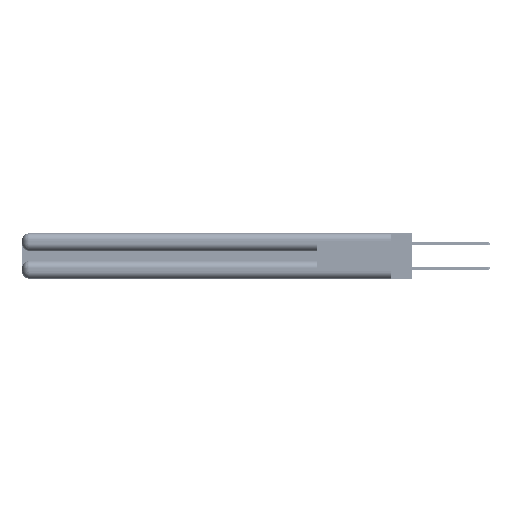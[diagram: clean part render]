
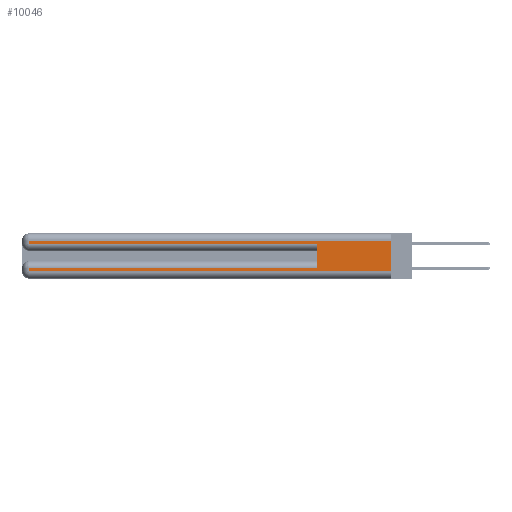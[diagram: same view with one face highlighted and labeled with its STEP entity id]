
A CAD part, left-side view. The second image highlights one B-rep face of the part: STEP entity #10046.
In plain terms, the highlighted planar face has unit normal (-1, 0, 0).
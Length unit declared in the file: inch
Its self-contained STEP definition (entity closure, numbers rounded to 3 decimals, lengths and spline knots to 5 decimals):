
#1455 = VERTEX_POINT ( 'NONE', #49478 ) ;
#1917 = DIRECTION ( 'NONE',  ( 0., 1., 0. ) ) ;
#2468 = CARTESIAN_POINT ( 'NONE',  ( 0., 0.6, 0.285 ) ) ;
#3749 = ORIENTED_EDGE ( 'NONE', *, *, #15448, .T. ) ;
#4022 = VECTOR ( 'NONE', #41665, 39.37008 ) ;
#4576 = EDGE_CURVE ( 'NONE', #1455, #8995, #44845, .T. ) ;
#5331 = LINE ( 'NONE', #37475, #4022 ) ;
#8507 = CARTESIAN_POINT ( 'NONE',  ( 0., 0., 0.06 ) ) ;
#8995 = VERTEX_POINT ( 'NONE', #20734 ) ;
#10046 = ADVANCED_FACE ( 'NONE', ( #35135 ), #47172, .F. ) ;
#10300 = ORIENTED_EDGE ( 'NONE', *, *, #4576, .T. ) ;
#10447 = DIRECTION ( 'NONE',  ( 0., 0., -1. ) ) ;
#10499 = EDGE_CURVE ( 'NONE', #41101, #53403, #35088, .T. ) ;
#13722 = ORIENTED_EDGE ( 'NONE', *, *, #42557, .T. ) ;
#13946 = CARTESIAN_POINT ( 'NONE',  ( 0., 0., 0.37 ) ) ;
#15448 = EDGE_CURVE ( 'NONE', #8995, #31490, #26411, .T. ) ;
#15453 = LINE ( 'NONE', #51748, #36203 ) ;
#15523 = EDGE_CURVE ( 'NONE', #40094, #53403, #23778, .T. ) ;
#15532 = ORIENTED_EDGE ( 'NONE', *, *, #18453, .T. ) ;
#16401 = CARTESIAN_POINT ( 'NONE',  ( 0., 0., 0.06 ) ) ;
#16631 = DIRECTION ( 'NONE',  ( 0., 0., 1. ) ) ;
#17705 = VECTOR ( 'NONE', #43293, 39.37008 ) ;
#18238 = ORIENTED_EDGE ( 'NONE', *, *, #21304, .T. ) ;
#18453 = EDGE_CURVE ( 'NONE', #41101, #1455, #5331, .T. ) ;
#19496 = DIRECTION ( 'NONE',  ( 0., 0., -1. ) ) ;
#19573 = AXIS2_PLACEMENT_3D ( 'NONE', #13946, #22275, #51353 ) ;
#20734 = CARTESIAN_POINT ( 'NONE',  ( 0., 2.94, 0.06 ) ) ;
#21285 = ORIENTED_EDGE ( 'NONE', *, *, #10499, .F. ) ;
#21304 = EDGE_CURVE ( 'NONE', #40150, #36391, #15453, .T. ) ;
#22275 = DIRECTION ( 'NONE',  ( 1., 0., 0. ) ) ;
#22719 = VECTOR ( 'NONE', #16631, 39.37008 ) ;
#23778 = LINE ( 'NONE', #46273, #33566 ) ;
#26411 = LINE ( 'NONE', #8507, #47197 ) ;
#28663 = CARTESIAN_POINT ( 'NONE',  ( 0., 0., 0.31 ) ) ;
#31097 = EDGE_CURVE ( 'NONE', #40150, #31490, #41115, .T. ) ;
#31490 = VERTEX_POINT ( 'NONE', #16401 ) ;
#33396 = DIRECTION ( 'NONE',  ( 0., -1., 0. ) ) ;
#33566 = VECTOR ( 'NONE', #33767, 39.37008 ) ;
#33767 = DIRECTION ( 'NONE',  ( 0., -1., 0. ) ) ;
#35088 = LINE ( 'NONE', #41696, #22719 ) ;
#35097 = VECTOR ( 'NONE', #10447, 39.37008 ) ;
#35135 = FACE_OUTER_BOUND ( 'NONE', #52192, .T. ) ;
#35742 = VECTOR ( 'NONE', #19496, 39.37008 ) ;
#36009 = CARTESIAN_POINT ( 'NONE',  ( 0., 2.94, 0.37 ) ) ;
#36203 = VECTOR ( 'NONE', #1917, 39.37008 ) ;
#36391 = VERTEX_POINT ( 'NONE', #45367 ) ;
#37475 = CARTESIAN_POINT ( 'NONE',  ( 0., 0., 0.085 ) ) ;
#39116 = CARTESIAN_POINT ( 'NONE',  ( 0., 0., 0.37 ) ) ;
#39514 = CARTESIAN_POINT ( 'NONE',  ( 0., 2.94, 0.37 ) ) ;
#39666 = LINE ( 'NONE', #36009, #35742 ) ;
#40094 = VERTEX_POINT ( 'NONE', #40651 ) ;
#40150 = VERTEX_POINT ( 'NONE', #28663 ) ;
#40651 = CARTESIAN_POINT ( 'NONE',  ( 0., 2.94, 0.285 ) ) ;
#41101 = VERTEX_POINT ( 'NONE', #43417 ) ;
#41115 = LINE ( 'NONE', #39116, #17705 ) ;
#41665 = DIRECTION ( 'NONE',  ( 0., 1., 0. ) ) ;
#41696 = CARTESIAN_POINT ( 'NONE',  ( 0., 0.6, 0.145 ) ) ;
#42557 = EDGE_CURVE ( 'NONE', #36391, #40094, #39666, .T. ) ;
#43293 = DIRECTION ( 'NONE',  ( 0., 0., -1. ) ) ;
#43417 = CARTESIAN_POINT ( 'NONE',  ( 0., 0.6, 0.085 ) ) ;
#44845 = LINE ( 'NONE', #39514, #35097 ) ;
#45367 = CARTESIAN_POINT ( 'NONE',  ( 0., 2.94, 0.31 ) ) ;
#46273 = CARTESIAN_POINT ( 'NONE',  ( 0., 0., 0.285 ) ) ;
#46851 = ORIENTED_EDGE ( 'NONE', *, *, #15523, .T. ) ;
#47172 = PLANE ( 'NONE',  #19573 ) ;
#47197 = VECTOR ( 'NONE', #33396, 39.37008 ) ;
#49478 = CARTESIAN_POINT ( 'NONE',  ( 0., 2.94, 0.085 ) ) ;
#51353 = DIRECTION ( 'NONE',  ( 0., 0., -1. ) ) ;
#51748 = CARTESIAN_POINT ( 'NONE',  ( 0., 0., 0.31 ) ) ;
#52192 = EDGE_LOOP ( 'NONE', ( #52667, #18238, #13722, #46851, #21285, #15532, #10300, #3749 ) ) ;
#52667 = ORIENTED_EDGE ( 'NONE', *, *, #31097, .F. ) ;
#53403 = VERTEX_POINT ( 'NONE', #2468 ) ;
